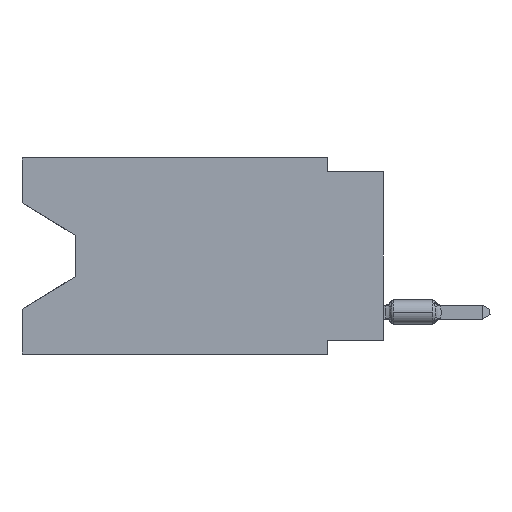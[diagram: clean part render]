
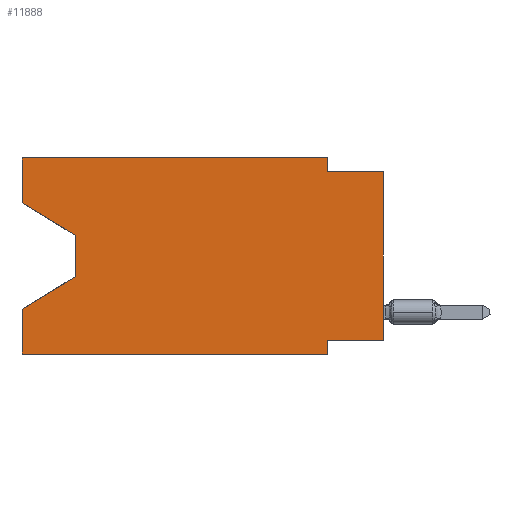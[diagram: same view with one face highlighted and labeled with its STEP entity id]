
A CAD part, left-side view. The second image highlights one B-rep face of the part: STEP entity #11888.
In plain terms, the highlighted planar face has unit normal (-1, 0, 0).
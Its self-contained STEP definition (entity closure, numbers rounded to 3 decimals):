
#30 = DIRECTION ( 'NONE',  ( 0., 0.855, -0.519 ) ) ;
#193 = DIRECTION ( 'NONE',  ( 0., -1., 0. ) ) ;
#678 = EDGE_CURVE ( 'NONE', #50852, #46408, #11746, .T. ) ;
#1290 = LINE ( 'NONE', #34512, #4268 ) ;
#1894 = DIRECTION ( 'NONE',  ( 0., 0., 1. ) ) ;
#2406 = ORIENTED_EDGE ( 'NONE', *, *, #20038, .F. ) ;
#3104 = CARTESIAN_POINT ( 'NONE',  ( 0., 2.54, -8.255 ) ) ;
#3692 = LINE ( 'NONE', #55523, #29313 ) ;
#4179 = VERTEX_POINT ( 'NONE', #34400 ) ;
#4268 = VECTOR ( 'NONE', #1894, 1000. ) ;
#4884 = VECTOR ( 'NONE', #51927, 1000. ) ;
#5244 = DIRECTION ( 'NONE',  ( 0., 0., -1. ) ) ;
#5561 = CARTESIAN_POINT ( 'NONE',  ( 0., 16.383, -8.89 ) ) ;
#6233 = ORIENTED_EDGE ( 'NONE', *, *, #37559, .T. ) ;
#6460 = CARTESIAN_POINT ( 'NONE',  ( 0., 0., 0. ) ) ;
#6931 = ORIENTED_EDGE ( 'NONE', *, *, #48607, .T. ) ;
#7344 = DIRECTION ( 'NONE',  ( 0., -1., 0. ) ) ;
#8387 = VERTEX_POINT ( 'NONE', #9394 ) ;
#8716 = VECTOR ( 'NONE', #52827, 1000. ) ;
#9070 = VERTEX_POINT ( 'NONE', #38925 ) ;
#9224 = DIRECTION ( 'NONE',  ( 0., 0., -1. ) ) ;
#9394 = CARTESIAN_POINT ( 'NONE',  ( 0., 2.54, -8.89 ) ) ;
#9855 = CARTESIAN_POINT ( 'NONE',  ( 0., 0., -8.255 ) ) ;
#10268 = VERTEX_POINT ( 'NONE', #47928 ) ;
#10416 = ORIENTED_EDGE ( 'NONE', *, *, #20043, .T. ) ;
#11317 = DIRECTION ( 'NONE',  ( 0., 0., 1. ) ) ;
#11386 = ORIENTED_EDGE ( 'NONE', *, *, #32298, .F. ) ;
#11746 = LINE ( 'NONE', #22092, #43804 ) ;
#11888 = ADVANCED_FACE ( 'NONE', ( #15900 ), #33898, .F. ) ;
#14553 = CARTESIAN_POINT ( 'NONE',  ( 0., 16.383, -2.038 ) ) ;
#14705 = VECTOR ( 'NONE', #45868, 1000. ) ;
#15900 = FACE_OUTER_BOUND ( 'NONE', #32608, .T. ) ;
#16167 = ORIENTED_EDGE ( 'NONE', *, *, #678, .T. ) ;
#17704 = CARTESIAN_POINT ( 'NONE',  ( 0., 0., -0.635 ) ) ;
#18139 = VERTEX_POINT ( 'NONE', #37123 ) ;
#19404 = VERTEX_POINT ( 'NONE', #49407 ) ;
#20038 = EDGE_CURVE ( 'NONE', #50852, #10268, #1290, .T. ) ;
#20043 = EDGE_CURVE ( 'NONE', #32677, #52338, #57994, .T. ) ;
#20136 = EDGE_CURVE ( 'NONE', #9070, #52338, #35698, .T. ) ;
#21277 = ORIENTED_EDGE ( 'NONE', *, *, #33511, .F. ) ;
#22092 = CARTESIAN_POINT ( 'NONE',  ( 0., 16.383, -2.038 ) ) ;
#22950 = CARTESIAN_POINT ( 'NONE',  ( 0., 2.54, -8.89 ) ) ;
#22961 = ORIENTED_EDGE ( 'NONE', *, *, #47205, .F. ) ;
#26793 = AXIS2_PLACEMENT_3D ( 'NONE', #51598, #47032, #5244 ) ;
#26798 = CARTESIAN_POINT ( 'NONE',  ( 0., 13.97, -3.505 ) ) ;
#27251 = LINE ( 'NONE', #53280, #14705 ) ;
#29313 = VECTOR ( 'NONE', #30, 1000. ) ;
#29339 = ORIENTED_EDGE ( 'NONE', *, *, #20136, .F. ) ;
#29765 = VERTEX_POINT ( 'NONE', #39146 ) ;
#30264 = VECTOR ( 'NONE', #9224, 1000. ) ;
#31470 = LINE ( 'NONE', #55250, #54550 ) ;
#32006 = ORIENTED_EDGE ( 'NONE', *, *, #48219, .F. ) ;
#32298 = EDGE_CURVE ( 'NONE', #19404, #9070, #31470, .T. ) ;
#32608 = EDGE_LOOP ( 'NONE', ( #16167, #47749, #6931, #22961, #6233, #32006, #21277, #10416, #29339, #11386, #60000, #2406 ) ) ;
#32677 = VERTEX_POINT ( 'NONE', #9855 ) ;
#32786 = LINE ( 'NONE', #45943, #44803 ) ;
#33511 = EDGE_CURVE ( 'NONE', #32677, #37866, #27251, .T. ) ;
#33898 = PLANE ( 'NONE',  #26793 ) ;
#34226 = CARTESIAN_POINT ( 'NONE',  ( 0., 16.383, 0. ) ) ;
#34279 = EDGE_CURVE ( 'NONE', #46408, #4179, #44503, .T. ) ;
#34400 = CARTESIAN_POINT ( 'NONE',  ( 0., 13.97, -5.385 ) ) ;
#34512 = CARTESIAN_POINT ( 'NONE',  ( 0., 16.383, 0. ) ) ;
#35698 = LINE ( 'NONE', #17704, #44187 ) ;
#36789 = VECTOR ( 'NONE', #54562, 1000. ) ;
#37123 = CARTESIAN_POINT ( 'NONE',  ( 0., 16.383, -6.852 ) ) ;
#37559 = EDGE_CURVE ( 'NONE', #29765, #8387, #47352, .T. ) ;
#37866 = VERTEX_POINT ( 'NONE', #3104 ) ;
#38925 = CARTESIAN_POINT ( 'NONE',  ( 0., 2.54, -0.635 ) ) ;
#39146 = CARTESIAN_POINT ( 'NONE',  ( 0., 16.383, -8.89 ) ) ;
#40445 = CARTESIAN_POINT ( 'NONE',  ( 0., 13.97, -3.505 ) ) ;
#40990 = LINE ( 'NONE', #22950, #30264 ) ;
#42557 = CARTESIAN_POINT ( 'NONE',  ( 0., 0., -0.635 ) ) ;
#43804 = VECTOR ( 'NONE', #58413, 1000. ) ;
#44187 = VECTOR ( 'NONE', #7344, 1000. ) ;
#44503 = LINE ( 'NONE', #26798, #36789 ) ;
#44803 = VECTOR ( 'NONE', #193, 1000. ) ;
#45868 = DIRECTION ( 'NONE',  ( 0., 1., 0. ) ) ;
#45943 = CARTESIAN_POINT ( 'NONE',  ( 0., 16.383, 0. ) ) ;
#46102 = DIRECTION ( 'NONE',  ( 0., 0., -1. ) ) ;
#46408 = VERTEX_POINT ( 'NONE', #40445 ) ;
#47032 = DIRECTION ( 'NONE',  ( 1., 0., 0. ) ) ;
#47205 = EDGE_CURVE ( 'NONE', #29765, #18139, #54839, .T. ) ;
#47352 = LINE ( 'NONE', #5561, #4884 ) ;
#47749 = ORIENTED_EDGE ( 'NONE', *, *, #34279, .T. ) ;
#47812 = EDGE_CURVE ( 'NONE', #10268, #19404, #32786, .T. ) ;
#47928 = CARTESIAN_POINT ( 'NONE',  ( 0., 16.383, 0. ) ) ;
#48219 = EDGE_CURVE ( 'NONE', #37866, #8387, #40990, .T. ) ;
#48607 = EDGE_CURVE ( 'NONE', #4179, #18139, #3692, .T. ) ;
#49407 = CARTESIAN_POINT ( 'NONE',  ( 0., 2.54, 0. ) ) ;
#50852 = VERTEX_POINT ( 'NONE', #14553 ) ;
#51598 = CARTESIAN_POINT ( 'NONE',  ( 0., 16.383, 0. ) ) ;
#51927 = DIRECTION ( 'NONE',  ( 0., -1., 0. ) ) ;
#52338 = VERTEX_POINT ( 'NONE', #42557 ) ;
#52827 = DIRECTION ( 'NONE',  ( 0., 0., 1. ) ) ;
#53280 = CARTESIAN_POINT ( 'NONE',  ( 0., 0., -8.255 ) ) ;
#54550 = VECTOR ( 'NONE', #46102, 1000. ) ;
#54562 = DIRECTION ( 'NONE',  ( 0., 0., -1. ) ) ;
#54839 = LINE ( 'NONE', #34226, #8716 ) ;
#55250 = CARTESIAN_POINT ( 'NONE',  ( 0., 2.54, 0. ) ) ;
#55523 = CARTESIAN_POINT ( 'NONE',  ( 0., 13.97, -5.385 ) ) ;
#55843 = VECTOR ( 'NONE', #11317, 1000. ) ;
#57994 = LINE ( 'NONE', #6460, #55843 ) ;
#58413 = DIRECTION ( 'NONE',  ( 0., -0.855, -0.519 ) ) ;
#60000 = ORIENTED_EDGE ( 'NONE', *, *, #47812, .F. ) ;
